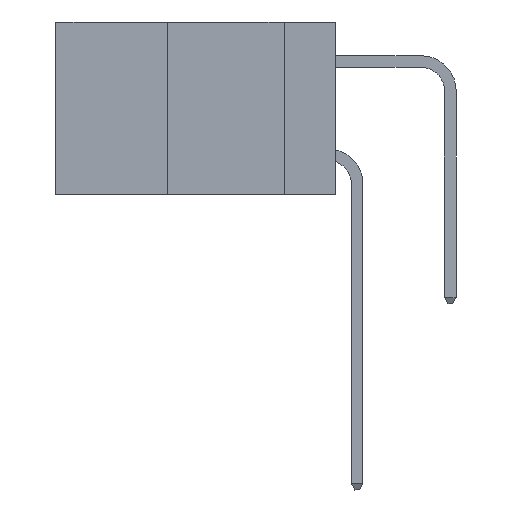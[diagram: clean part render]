
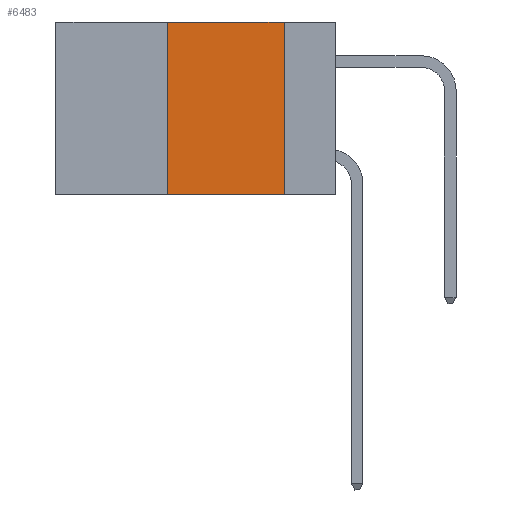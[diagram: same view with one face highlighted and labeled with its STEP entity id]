
A CAD part, left-side view. The second image highlights one B-rep face of the part: STEP entity #6483.
In plain terms, the highlighted planar face has unit normal (-1, 0, 0).
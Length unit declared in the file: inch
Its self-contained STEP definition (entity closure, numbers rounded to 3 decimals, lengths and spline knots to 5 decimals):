
#1328 = CARTESIAN_POINT ( 'NONE',  ( 0., 0.11, 0. ) ) ;
#1938 = ORIENTED_EDGE ( 'NONE', *, *, #2751, .F. ) ;
#2299 = LINE ( 'NONE', #24596, #22605 ) ;
#2751 = EDGE_CURVE ( 'NONE', #7816, #5013, #2967, .T. ) ;
#2803 = DIRECTION ( 'NONE',  ( 0., 0., 1. ) ) ;
#2967 = LINE ( 'NONE', #20203, #12934 ) ;
#4853 = VERTEX_POINT ( 'NONE', #14755 ) ;
#5013 = VERTEX_POINT ( 'NONE', #1328 ) ;
#5153 = VECTOR ( 'NONE', #20617, 39.37008 ) ;
#6035 = DIRECTION ( 'NONE',  ( 1., 0., 0. ) ) ;
#6248 = FACE_OUTER_BOUND ( 'NONE', #8852, .T. ) ;
#6483 = ADVANCED_FACE ( 'NONE', ( #6248 ), #13900, .F. ) ;
#7816 = VERTEX_POINT ( 'NONE', #23210 ) ;
#8852 = EDGE_LOOP ( 'NONE', ( #21672, #1938, #18368, #10097 ) ) ;
#9405 = AXIS2_PLACEMENT_3D ( 'NONE', #11895, #6035, #19754 ) ;
#10097 = ORIENTED_EDGE ( 'NONE', *, *, #22767, .T. ) ;
#11895 = CARTESIAN_POINT ( 'NONE',  ( 0., 0.6, 0. ) ) ;
#12879 = CARTESIAN_POINT ( 'NONE',  ( 0., 0.6, -0.37 ) ) ;
#12934 = VECTOR ( 'NONE', #22148, 39.37008 ) ;
#13190 = EDGE_CURVE ( 'NONE', #20223, #7816, #22652, .T. ) ;
#13900 = PLANE ( 'NONE',  #9405 ) ;
#14025 = EDGE_CURVE ( 'NONE', #5013, #4853, #2299, .T. ) ;
#14755 = CARTESIAN_POINT ( 'NONE',  ( 0., 0.11, -0.37 ) ) ;
#15009 = DIRECTION ( 'NONE',  ( 0., 0., -1. ) ) ;
#18368 = ORIENTED_EDGE ( 'NONE', *, *, #13190, .F. ) ;
#19754 = DIRECTION ( 'NONE',  ( 0., 0., -1. ) ) ;
#20019 = CARTESIAN_POINT ( 'NONE',  ( 0., 0.36, -0.37 ) ) ;
#20203 = CARTESIAN_POINT ( 'NONE',  ( 0., 0.6, 0. ) ) ;
#20223 = VERTEX_POINT ( 'NONE', #20019 ) ;
#20464 = CARTESIAN_POINT ( 'NONE',  ( 0., 0.36, 0. ) ) ;
#20617 = DIRECTION ( 'NONE',  ( 0., -1., 0. ) ) ;
#20811 = LINE ( 'NONE', #12879, #5153 ) ;
#21451 = VECTOR ( 'NONE', #2803, 39.37008 ) ;
#21672 = ORIENTED_EDGE ( 'NONE', *, *, #14025, .F. ) ;
#22148 = DIRECTION ( 'NONE',  ( 0., -1., 0. ) ) ;
#22605 = VECTOR ( 'NONE', #15009, 39.37008 ) ;
#22652 = LINE ( 'NONE', #20464, #21451 ) ;
#22767 = EDGE_CURVE ( 'NONE', #20223, #4853, #20811, .T. ) ;
#23210 = CARTESIAN_POINT ( 'NONE',  ( 0., 0.36, 0. ) ) ;
#24596 = CARTESIAN_POINT ( 'NONE',  ( 0., 0.11, 0. ) ) ;
